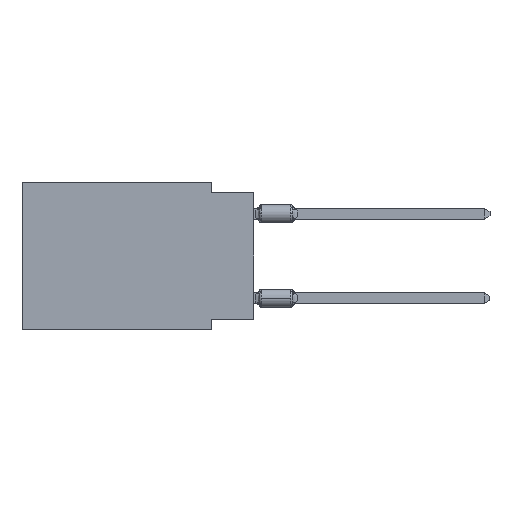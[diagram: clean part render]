
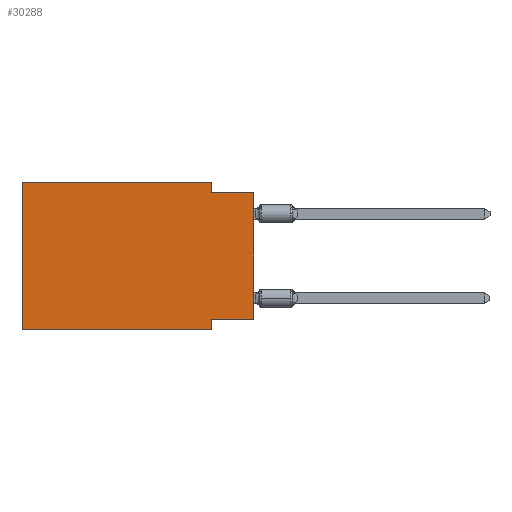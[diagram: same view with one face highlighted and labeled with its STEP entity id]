
A CAD part, left-side view. The second image highlights one B-rep face of the part: STEP entity #30288.
In plain terms, the highlighted planar face has unit normal (-1, 0, 0).
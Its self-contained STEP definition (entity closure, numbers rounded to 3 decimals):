
#295 = CARTESIAN_POINT ( 'NONE',  ( 0., 13.97, -8.89 ) ) ;
#529 = CARTESIAN_POINT ( 'NONE',  ( 0., 2.54, -8.255 ) ) ;
#944 = CARTESIAN_POINT ( 'NONE',  ( 0., 2.54, -0.635 ) ) ;
#1805 = ORIENTED_EDGE ( 'NONE', *, *, #17279, .F. ) ;
#2687 = ORIENTED_EDGE ( 'NONE', *, *, #29771, .T. ) ;
#2751 = EDGE_CURVE ( 'NONE', #24350, #24675, #26310, .T. ) ;
#3460 = ORIENTED_EDGE ( 'NONE', *, *, #15688, .F. ) ;
#3511 = CARTESIAN_POINT ( 'NONE',  ( 0., 2.54, 0. ) ) ;
#3744 = LINE ( 'NONE', #3894, #4236 ) ;
#3759 = DIRECTION ( 'NONE',  ( 1., 0., 0. ) ) ;
#3894 = CARTESIAN_POINT ( 'NONE',  ( 0., 0., -8.255 ) ) ;
#4079 = EDGE_CURVE ( 'NONE', #9515, #24675, #8450, .T. ) ;
#4236 = VECTOR ( 'NONE', #10988, 1000. ) ;
#4338 = LINE ( 'NONE', #23301, #8752 ) ;
#4479 = LINE ( 'NONE', #23290, #27815 ) ;
#6601 = CARTESIAN_POINT ( 'NONE',  ( 0., 0., -0.635 ) ) ;
#8043 = VERTEX_POINT ( 'NONE', #9249 ) ;
#8191 = CARTESIAN_POINT ( 'NONE',  ( 0., 13.97, 0. ) ) ;
#8256 = CARTESIAN_POINT ( 'NONE',  ( 0., 13.97, -8.89 ) ) ;
#8450 = LINE ( 'NONE', #26802, #25742 ) ;
#8689 = VECTOR ( 'NONE', #28089, 1000. ) ;
#8752 = VECTOR ( 'NONE', #20379, 1000. ) ;
#9065 = CARTESIAN_POINT ( 'NONE',  ( 0., 2.54, -8.89 ) ) ;
#9249 = CARTESIAN_POINT ( 'NONE',  ( 0., 13.97, 0. ) ) ;
#9353 = VERTEX_POINT ( 'NONE', #11484 ) ;
#9515 = VERTEX_POINT ( 'NONE', #529 ) ;
#10062 = VERTEX_POINT ( 'NONE', #944 ) ;
#10356 = DIRECTION ( 'NONE',  ( 0., 0., 1. ) ) ;
#10680 = EDGE_LOOP ( 'NONE', ( #2687, #24587, #23257, #3460, #1805, #17842, #24897, #17027 ) ) ;
#10815 = LINE ( 'NONE', #8191, #26051 ) ;
#10988 = DIRECTION ( 'NONE',  ( 0., 1., 0. ) ) ;
#11484 = CARTESIAN_POINT ( 'NONE',  ( 0., 0., -8.255 ) ) ;
#12916 = DIRECTION ( 'NONE',  ( 0., 0., -1. ) ) ;
#13144 = EDGE_CURVE ( 'NONE', #10062, #14568, #30045, .T. ) ;
#14027 = DIRECTION ( 'NONE',  ( 0., 0., 1. ) ) ;
#14568 = VERTEX_POINT ( 'NONE', #20528 ) ;
#15484 = FACE_OUTER_BOUND ( 'NONE', #10680, .T. ) ;
#15688 = EDGE_CURVE ( 'NONE', #8043, #27593, #4338, .T. ) ;
#17027 = ORIENTED_EDGE ( 'NONE', *, *, #26807, .F. ) ;
#17279 = EDGE_CURVE ( 'NONE', #24350, #8043, #10815, .T. ) ;
#17647 = PLANE ( 'NONE',  #29297 ) ;
#17842 = ORIENTED_EDGE ( 'NONE', *, *, #2751, .T. ) ;
#18202 = VECTOR ( 'NONE', #25441, 1000. ) ;
#18981 = LINE ( 'NONE', #19135, #8689 ) ;
#19135 = CARTESIAN_POINT ( 'NONE',  ( 0., 2.54, 0. ) ) ;
#19806 = DIRECTION ( 'NONE',  ( 0., 0., -1. ) ) ;
#19867 = VECTOR ( 'NONE', #29677, 1000. ) ;
#20379 = DIRECTION ( 'NONE',  ( 0., -1., 0. ) ) ;
#20528 = CARTESIAN_POINT ( 'NONE',  ( 0., 0., -0.635 ) ) ;
#23257 = ORIENTED_EDGE ( 'NONE', *, *, #26915, .F. ) ;
#23290 = CARTESIAN_POINT ( 'NONE',  ( 0., 0., 0. ) ) ;
#23301 = CARTESIAN_POINT ( 'NONE',  ( 0., 13.97, 0. ) ) ;
#24350 = VERTEX_POINT ( 'NONE', #295 ) ;
#24587 = ORIENTED_EDGE ( 'NONE', *, *, #13144, .F. ) ;
#24675 = VERTEX_POINT ( 'NONE', #9065 ) ;
#24897 = ORIENTED_EDGE ( 'NONE', *, *, #4079, .F. ) ;
#25441 = DIRECTION ( 'NONE',  ( 0., -1., 0. ) ) ;
#25742 = VECTOR ( 'NONE', #12916, 1000. ) ;
#26051 = VECTOR ( 'NONE', #10356, 1000. ) ;
#26310 = LINE ( 'NONE', #8256, #19867 ) ;
#26802 = CARTESIAN_POINT ( 'NONE',  ( 0., 2.54, -8.89 ) ) ;
#26807 = EDGE_CURVE ( 'NONE', #9353, #9515, #3744, .T. ) ;
#26915 = EDGE_CURVE ( 'NONE', #27593, #10062, #18981, .T. ) ;
#27593 = VERTEX_POINT ( 'NONE', #3511 ) ;
#27815 = VECTOR ( 'NONE', #14027, 1000. ) ;
#28089 = DIRECTION ( 'NONE',  ( 0., 0., -1. ) ) ;
#29297 = AXIS2_PLACEMENT_3D ( 'NONE', #29658, #3759, #19806 ) ;
#29658 = CARTESIAN_POINT ( 'NONE',  ( 0., 13.97, 0. ) ) ;
#29677 = DIRECTION ( 'NONE',  ( 0., -1., 0. ) ) ;
#29771 = EDGE_CURVE ( 'NONE', #9353, #14568, #4479, .T. ) ;
#30045 = LINE ( 'NONE', #6601, #18202 ) ;
#30288 = ADVANCED_FACE ( 'NONE', ( #15484 ), #17647, .F. ) ;
